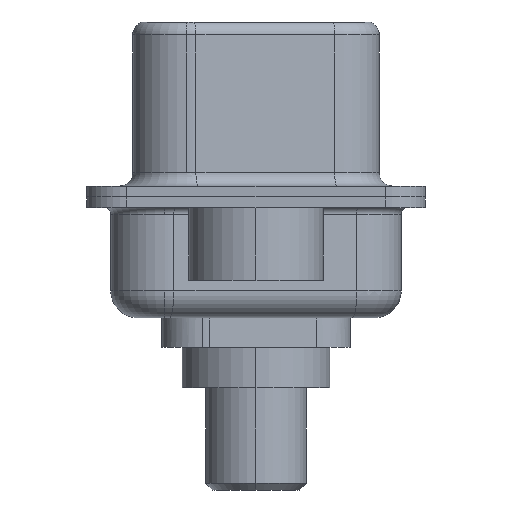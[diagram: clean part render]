
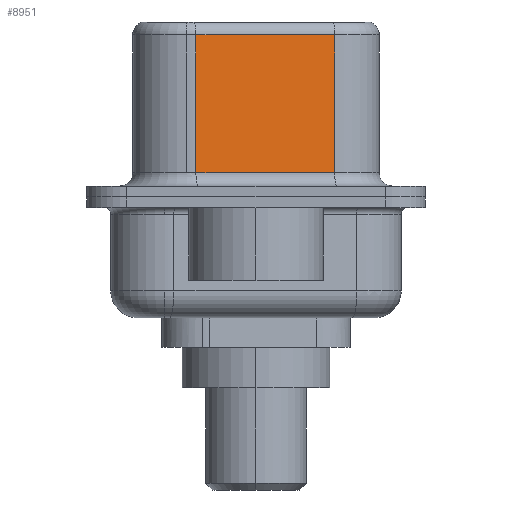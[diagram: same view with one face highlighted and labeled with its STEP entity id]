
A CAD part, left-side view. The second image highlights one B-rep face of the part: STEP entity #8951.
In plain terms, the highlighted planar face has unit normal (-0.985, -0.174, 0).
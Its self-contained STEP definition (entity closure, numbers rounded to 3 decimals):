
#845 = DIRECTION ( 'NONE',  ( 0.985, 0.174, 0. ) ) ;
#1810 = DIRECTION ( 'NONE',  ( 0., 0., -1. ) ) ;
#1864 = CARTESIAN_POINT ( 'NONE',  ( 3.67, 2.233, 6.02 ) ) ;
#2196 = FACE_OUTER_BOUND ( 'NONE', #8525, .T. ) ;
#2577 = ORIENTED_EDGE ( 'NONE', *, *, #13419, .T. ) ;
#3361 = LINE ( 'NONE', #8310, #14487 ) ;
#3591 = VECTOR ( 'NONE', #12909, 1000. ) ;
#3935 = LINE ( 'NONE', #14071, #16438 ) ;
#4776 = LINE ( 'NONE', #10130, #14690 ) ;
#7101 = VERTEX_POINT ( 'NONE', #11865 ) ;
#7905 = AXIS2_PLACEMENT_3D ( 'NONE', #12581, #845, #9983 ) ;
#8228 = EDGE_CURVE ( 'NONE', #11321, #10667, #3935, .T. ) ;
#8274 = CARTESIAN_POINT ( 'NONE',  ( 4.58, -2.927, 0.9 ) ) ;
#8310 = CARTESIAN_POINT ( 'NONE',  ( 4.58, -2.927, 6.52 ) ) ;
#8525 = EDGE_LOOP ( 'NONE', ( #13186, #14123, #11421, #2577 ) ) ;
#8892 = CARTESIAN_POINT ( 'NONE',  ( 4.58, -2.927, 6.02 ) ) ;
#8951 = ADVANCED_FACE ( 'NONE', ( #2196 ), #13778, .F. ) ;
#9587 = VERTEX_POINT ( 'NONE', #8274 ) ;
#9983 = DIRECTION ( 'NONE',  ( -0.174, 0.985, 0. ) ) ;
#10109 = DIRECTION ( 'NONE',  ( 0., 0., -1. ) ) ;
#10130 = CARTESIAN_POINT ( 'NONE',  ( 4.58, -2.927, 0.9 ) ) ;
#10399 = LINE ( 'NONE', #8892, #3591 ) ;
#10667 = VERTEX_POINT ( 'NONE', #11642 ) ;
#11321 = VERTEX_POINT ( 'NONE', #1864 ) ;
#11421 = ORIENTED_EDGE ( 'NONE', *, *, #8228, .T. ) ;
#11642 = CARTESIAN_POINT ( 'NONE',  ( 3.67, 2.233, 0.9 ) ) ;
#11865 = CARTESIAN_POINT ( 'NONE',  ( 4.58, -2.927, 6.02 ) ) ;
#12581 = CARTESIAN_POINT ( 'NONE',  ( 4.58, -2.927, 6.52 ) ) ;
#12909 = DIRECTION ( 'NONE',  ( -0.174, 0.985, 0. ) ) ;
#13186 = ORIENTED_EDGE ( 'NONE', *, *, #13822, .F. ) ;
#13419 = EDGE_CURVE ( 'NONE', #10667, #9587, #4776, .T. ) ;
#13479 = EDGE_CURVE ( 'NONE', #7101, #11321, #10399, .T. ) ;
#13778 = PLANE ( 'NONE',  #7905 ) ;
#13822 = EDGE_CURVE ( 'NONE', #7101, #9587, #3361, .T. ) ;
#14071 = CARTESIAN_POINT ( 'NONE',  ( 3.67, 2.233, 6.52 ) ) ;
#14123 = ORIENTED_EDGE ( 'NONE', *, *, #13479, .T. ) ;
#14487 = VECTOR ( 'NONE', #1810, 1000. ) ;
#14690 = VECTOR ( 'NONE', #15326, 1000. ) ;
#15326 = DIRECTION ( 'NONE',  ( 0.174, -0.985, 0. ) ) ;
#16438 = VECTOR ( 'NONE', #10109, 1000. ) ;
